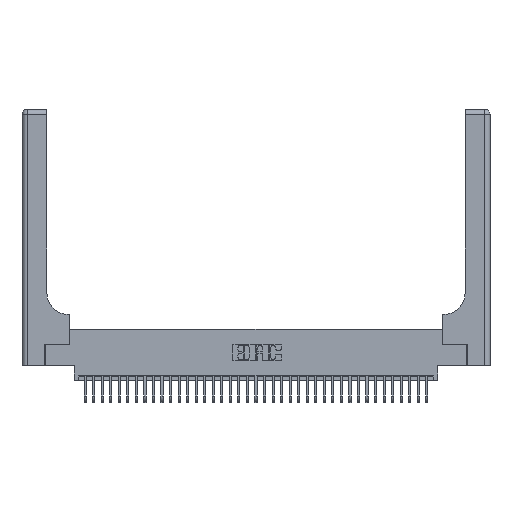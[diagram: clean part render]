
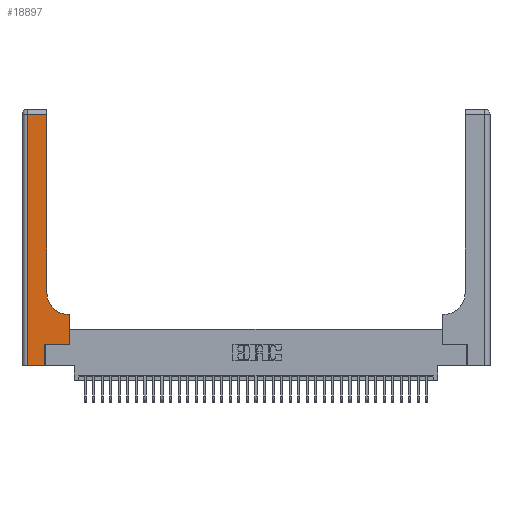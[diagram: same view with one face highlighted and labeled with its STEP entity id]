
A CAD part, top view. The second image highlights one B-rep face of the part: STEP entity #18897.
In plain terms, the highlighted planar face has unit normal (0, 0, 1).
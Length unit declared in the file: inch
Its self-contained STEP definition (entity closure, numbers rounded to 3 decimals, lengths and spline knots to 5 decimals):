
#595 = CARTESIAN_POINT ( 'NONE',  ( 0., 2.94, 0.37 ) ) ;
#915 = LINE ( 'NONE', #23561, #17174 ) ;
#1078 = CARTESIAN_POINT ( 'NONE',  ( 0.2915, 2.94, 0.37 ) ) ;
#1390 = DIRECTION ( 'NONE',  ( -1., 0., 0. ) ) ;
#2251 = DIRECTION ( 'NONE',  ( 0., -1., 0. ) ) ;
#2262 = CARTESIAN_POINT ( 'NONE',  ( 0.269, 0., 0.37 ) ) ;
#2630 = CARTESIAN_POINT ( 'NONE',  ( 0.5415, 0.6, 0.37 ) ) ;
#2887 = ORIENTED_EDGE ( 'NONE', *, *, #3925, .T. ) ;
#3925 = EDGE_CURVE ( 'NONE', #5432, #19213, #915, .T. ) ;
#4953 = AXIS2_PLACEMENT_3D ( 'NONE', #34707, #7426, #1390 ) ;
#5333 = EDGE_CURVE ( 'NONE', #31190, #26089, #26971, .T. ) ;
#5432 = VERTEX_POINT ( 'NONE', #17102 ) ;
#5603 = CARTESIAN_POINT ( 'NONE',  ( 0.5585, 0.6, 0.37 ) ) ;
#7089 = CARTESIAN_POINT ( 'NONE',  ( 0.269, 0., 0.37 ) ) ;
#7181 = LINE ( 'NONE', #7089, #36556 ) ;
#7426 = DIRECTION ( 'NONE',  ( 0., 0., -1. ) ) ;
#7704 = ORIENTED_EDGE ( 'NONE', *, *, #20466, .T. ) ;
#8209 = CARTESIAN_POINT ( 'NONE',  ( 0.5415, 0.85, 0.37 ) ) ;
#8561 = EDGE_CURVE ( 'NONE', #33972, #16724, #7181, .T. ) ;
#9625 = ORIENTED_EDGE ( 'NONE', *, *, #11314, .T. ) ;
#10287 = DIRECTION ( 'NONE',  ( 0., 1., 0. ) ) ;
#10308 = VECTOR ( 'NONE', #18912, 39.37008 ) ;
#10538 = VERTEX_POINT ( 'NONE', #2630 ) ;
#10752 = CARTESIAN_POINT ( 'NONE',  ( 0.269, 0.25, 0.37 ) ) ;
#11073 = AXIS2_PLACEMENT_3D ( 'NONE', #8209, #29436, #11270 ) ;
#11270 = DIRECTION ( 'NONE',  ( 1., 0., 0. ) ) ;
#11314 = EDGE_CURVE ( 'NONE', #36461, #10538, #23648, .T. ) ;
#11347 = VECTOR ( 'NONE', #19967, 39.37008 ) ;
#11558 = EDGE_LOOP ( 'NONE', ( #24325, #17247, #2887, #11972, #38015, #14825, #7704, #9625, #33790 ) ) ;
#11972 = ORIENTED_EDGE ( 'NONE', *, *, #34329, .T. ) ;
#13619 = CARTESIAN_POINT ( 'NONE',  ( 0., 0., 0.37 ) ) ;
#14825 = ORIENTED_EDGE ( 'NONE', *, *, #19504, .T. ) ;
#16565 = LINE ( 'NONE', #13619, #37797 ) ;
#16724 = VERTEX_POINT ( 'NONE', #10752 ) ;
#16911 = CARTESIAN_POINT ( 'NONE',  ( 0.5585, 0.25, 0.37 ) ) ;
#17102 = CARTESIAN_POINT ( 'NONE',  ( 0.06, 2.94, 0.37 ) ) ;
#17174 = VECTOR ( 'NONE', #2251, 39.37008 ) ;
#17247 = ORIENTED_EDGE ( 'NONE', *, *, #18777, .T. ) ;
#18777 = EDGE_CURVE ( 'NONE', #26089, #5432, #26441, .T. ) ;
#18897 = ADVANCED_FACE ( 'NONE', ( #38688 ), #37751, .F. ) ;
#18912 = DIRECTION ( 'NONE',  ( -1., 0., 0. ) ) ;
#19032 = EDGE_CURVE ( 'NONE', #10538, #31190, #35377, .T. ) ;
#19213 = VERTEX_POINT ( 'NONE', #30359 ) ;
#19504 = EDGE_CURVE ( 'NONE', #16724, #28006, #37485, .T. ) ;
#19967 = DIRECTION ( 'NONE',  ( 0., 1., 0. ) ) ;
#20035 = CARTESIAN_POINT ( 'NONE',  ( 0.5585, 0.25, 0.37 ) ) ;
#20466 = EDGE_CURVE ( 'NONE', #28006, #36461, #35497, .T. ) ;
#20488 = VECTOR ( 'NONE', #36909, 39.37008 ) ;
#22715 = VECTOR ( 'NONE', #24294, 39.37008 ) ;
#23561 = CARTESIAN_POINT ( 'NONE',  ( 0.06, 3., 0.37 ) ) ;
#23648 = LINE ( 'NONE', #36296, #22715 ) ;
#24294 = DIRECTION ( 'NONE',  ( -1., 0., 0. ) ) ;
#24325 = ORIENTED_EDGE ( 'NONE', *, *, #5333, .T. ) ;
#26089 = VERTEX_POINT ( 'NONE', #1078 ) ;
#26441 = LINE ( 'NONE', #595, #10308 ) ;
#26971 = LINE ( 'NONE', #34773, #39230 ) ;
#28006 = VERTEX_POINT ( 'NONE', #20035 ) ;
#29436 = DIRECTION ( 'NONE',  ( 0., 0., -1. ) ) ;
#30359 = CARTESIAN_POINT ( 'NONE',  ( 0.06, 0., 0.37 ) ) ;
#31190 = VERTEX_POINT ( 'NONE', #31709 ) ;
#31709 = CARTESIAN_POINT ( 'NONE',  ( 0.2915, 0.85, 0.37 ) ) ;
#33790 = ORIENTED_EDGE ( 'NONE', *, *, #19032, .T. ) ;
#33861 = CARTESIAN_POINT ( 'NONE',  ( 0.269, 0.25, 0.37 ) ) ;
#33972 = VERTEX_POINT ( 'NONE', #2262 ) ;
#34329 = EDGE_CURVE ( 'NONE', #19213, #33972, #16565, .T. ) ;
#34707 = CARTESIAN_POINT ( 'NONE',  ( 0., 3., 0.37 ) ) ;
#34773 = CARTESIAN_POINT ( 'NONE',  ( 0.2915, 3., 0.37 ) ) ;
#35377 = CIRCLE ( 'NONE', #11073, 0.25 ) ;
#35497 = LINE ( 'NONE', #16911, #11347 ) ;
#36296 = CARTESIAN_POINT ( 'NONE',  ( 0.2915, 0.6, 0.37 ) ) ;
#36461 = VERTEX_POINT ( 'NONE', #5603 ) ;
#36556 = VECTOR ( 'NONE', #10287, 39.37008 ) ;
#36909 = DIRECTION ( 'NONE',  ( 1., 0., 0. ) ) ;
#37485 = LINE ( 'NONE', #33861, #20488 ) ;
#37751 = PLANE ( 'NONE',  #4953 ) ;
#37797 = VECTOR ( 'NONE', #37832, 39.37008 ) ;
#37818 = DIRECTION ( 'NONE',  ( 0., 1., 0. ) ) ;
#37832 = DIRECTION ( 'NONE',  ( 1., 0., 0. ) ) ;
#38015 = ORIENTED_EDGE ( 'NONE', *, *, #8561, .T. ) ;
#38688 = FACE_OUTER_BOUND ( 'NONE', #11558, .T. ) ;
#39230 = VECTOR ( 'NONE', #37818, 39.37008 ) ;
